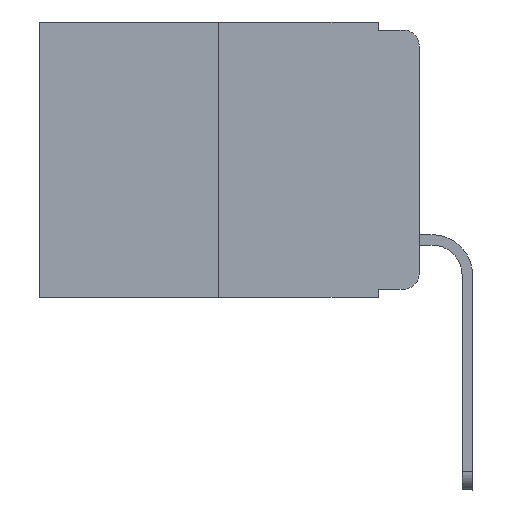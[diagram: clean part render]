
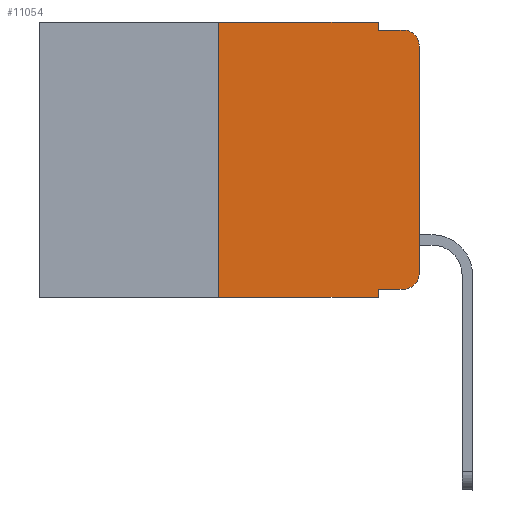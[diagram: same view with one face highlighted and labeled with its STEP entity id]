
A CAD part, left-side view. The second image highlights one B-rep face of the part: STEP entity #11054.
In plain terms, the highlighted planar face has unit normal (-1, 0, 0).
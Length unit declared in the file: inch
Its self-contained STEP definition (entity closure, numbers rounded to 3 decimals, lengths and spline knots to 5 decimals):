
#347 = CARTESIAN_POINT ( 'NONE',  ( 0., 0.051, -0.01 ) ) ;
#388 = CARTESIAN_POINT ( 'NONE',  ( 0., 0.473, 0. ) ) ;
#675 = EDGE_CURVE ( 'NONE', #12821, #10459, #7891, .T. ) ;
#1266 = CARTESIAN_POINT ( 'NONE',  ( 0., 0.051, 0. ) ) ;
#1323 = VERTEX_POINT ( 'NONE', #13808 ) ;
#1565 = DIRECTION ( 'NONE',  ( 0., -1., 0. ) ) ;
#1709 = CARTESIAN_POINT ( 'NONE',  ( 0., 0.051, 0. ) ) ;
#1970 = CARTESIAN_POINT ( 'NONE',  ( 0., 0.051, -0.01 ) ) ;
#2154 = EDGE_CURVE ( 'NONE', #12821, #5917, #11791, .T. ) ;
#2220 = DIRECTION ( 'NONE',  ( 0., 0., 1. ) ) ;
#2489 = DIRECTION ( 'NONE',  ( 0., -1., 0. ) ) ;
#2566 = DIRECTION ( 'NONE',  ( -1., 0., 0. ) ) ;
#2672 = CIRCLE ( 'NONE', #10478, 0.02 ) ;
#2825 = VECTOR ( 'NONE', #4316, 39.37008 ) ;
#2851 = VECTOR ( 'NONE', #2489, 39.37008 ) ;
#2893 = VERTEX_POINT ( 'NONE', #7720 ) ;
#2899 = CARTESIAN_POINT ( 'NONE',  ( 0., 0.25, -0.343 ) ) ;
#2956 = CIRCLE ( 'NONE', #10299, 0.02 ) ;
#3378 = CARTESIAN_POINT ( 'NONE',  ( 0., 0.25, 0. ) ) ;
#3440 = VECTOR ( 'NONE', #4258, 39.37008 ) ;
#3486 = VECTOR ( 'NONE', #8266, 39.37008 ) ;
#3659 = FACE_OUTER_BOUND ( 'NONE', #3898, .T. ) ;
#3717 = CARTESIAN_POINT ( 'NONE',  ( 0., 0.02, -0.03 ) ) ;
#3898 = EDGE_LOOP ( 'NONE', ( #11096, #4156, #4925, #9494, #6203, #8391, #6748, #5060, #5906, #5038 ) ) ;
#4055 = CARTESIAN_POINT ( 'NONE',  ( 0., 0.051, -0.333 ) ) ;
#4156 = ORIENTED_EDGE ( 'NONE', *, *, #6017, .T. ) ;
#4258 = DIRECTION ( 'NONE',  ( 0., 0., -1. ) ) ;
#4316 = DIRECTION ( 'NONE',  ( 0., -1., 0. ) ) ;
#4641 = LINE ( 'NONE', #388, #2851 ) ;
#4760 = DIRECTION ( 'NONE',  ( 0., 0., -1. ) ) ;
#4794 = DIRECTION ( 'NONE',  ( 0., 0., -1. ) ) ;
#4925 = ORIENTED_EDGE ( 'NONE', *, *, #9600, .F. ) ;
#4946 = VECTOR ( 'NONE', #1565, 39.37008 ) ;
#4984 = EDGE_CURVE ( 'NONE', #10326, #8712, #2672, .T. ) ;
#5018 = VECTOR ( 'NONE', #11070, 39.37008 ) ;
#5032 = CARTESIAN_POINT ( 'NONE',  ( 0., 0.473, -0.343 ) ) ;
#5038 = ORIENTED_EDGE ( 'NONE', *, *, #4984, .T. ) ;
#5060 = ORIENTED_EDGE ( 'NONE', *, *, #6753, .F. ) ;
#5211 = VERTEX_POINT ( 'NONE', #1709 ) ;
#5230 = CARTESIAN_POINT ( 'NONE',  ( 0., 0., 0. ) ) ;
#5351 = CARTESIAN_POINT ( 'NONE',  ( 0., 0.02, -0.313 ) ) ;
#5906 = ORIENTED_EDGE ( 'NONE', *, *, #10323, .T. ) ;
#5917 = VERTEX_POINT ( 'NONE', #8005 ) ;
#6017 = EDGE_CURVE ( 'NONE', #2893, #10927, #2956, .T. ) ;
#6203 = ORIENTED_EDGE ( 'NONE', *, *, #11391, .F. ) ;
#6416 = VECTOR ( 'NONE', #4760, 39.37008 ) ;
#6748 = ORIENTED_EDGE ( 'NONE', *, *, #2154, .T. ) ;
#6753 = EDGE_CURVE ( 'NONE', #1323, #5917, #13077, .T. ) ;
#6872 = EDGE_CURVE ( 'NONE', #5211, #7690, #12439, .T. ) ;
#6873 = DIRECTION ( 'NONE',  ( 1., 0., 0. ) ) ;
#7190 = LINE ( 'NONE', #1970, #3486 ) ;
#7275 = CARTESIAN_POINT ( 'NONE',  ( 0., 0.02, -0.333 ) ) ;
#7384 = LINE ( 'NONE', #5230, #10668 ) ;
#7690 = VERTEX_POINT ( 'NONE', #347 ) ;
#7720 = CARTESIAN_POINT ( 'NONE',  ( 0., 0., -0.03 ) ) ;
#7891 = LINE ( 'NONE', #13551, #5018 ) ;
#8005 = CARTESIAN_POINT ( 'NONE',  ( 0., 0.051, -0.343 ) ) ;
#8129 = CARTESIAN_POINT ( 'NONE',  ( 0., 0.051, 0. ) ) ;
#8266 = DIRECTION ( 'NONE',  ( 0., -1., 0. ) ) ;
#8391 = ORIENTED_EDGE ( 'NONE', *, *, #675, .F. ) ;
#8712 = VERTEX_POINT ( 'NONE', #12543 ) ;
#9049 = PLANE ( 'NONE',  #13811 ) ;
#9090 = DIRECTION ( 'NONE',  ( -1., 0., 0. ) ) ;
#9494 = ORIENTED_EDGE ( 'NONE', *, *, #6872, .F. ) ;
#9600 = EDGE_CURVE ( 'NONE', #7690, #10927, #7190, .T. ) ;
#10090 = DIRECTION ( 'NONE',  ( 0., 0., -1. ) ) ;
#10129 = DIRECTION ( 'NONE',  ( 0., 0., -1. ) ) ;
#10299 = AXIS2_PLACEMENT_3D ( 'NONE', #3717, #2566, #4794 ) ;
#10323 = EDGE_CURVE ( 'NONE', #1323, #10326, #13850, .T. ) ;
#10326 = VERTEX_POINT ( 'NONE', #7275 ) ;
#10459 = VERTEX_POINT ( 'NONE', #3378 ) ;
#10478 = AXIS2_PLACEMENT_3D ( 'NONE', #5351, #9090, #10090 ) ;
#10668 = VECTOR ( 'NONE', #2220, 39.37008 ) ;
#10927 = VERTEX_POINT ( 'NONE', #13129 ) ;
#11054 = ADVANCED_FACE ( 'NONE', ( #3659 ), #9049, .F. ) ;
#11070 = DIRECTION ( 'NONE',  ( 0., 0., 1. ) ) ;
#11096 = ORIENTED_EDGE ( 'NONE', *, *, #13478, .T. ) ;
#11391 = EDGE_CURVE ( 'NONE', #10459, #5211, #4641, .T. ) ;
#11791 = LINE ( 'NONE', #5032, #4946 ) ;
#12439 = LINE ( 'NONE', #8129, #6416 ) ;
#12543 = CARTESIAN_POINT ( 'NONE',  ( 0., 0., -0.313 ) ) ;
#12821 = VERTEX_POINT ( 'NONE', #2899 ) ;
#13077 = LINE ( 'NONE', #1266, #3440 ) ;
#13129 = CARTESIAN_POINT ( 'NONE',  ( 0., 0.02, -0.01 ) ) ;
#13478 = EDGE_CURVE ( 'NONE', #8712, #2893, #7384, .T. ) ;
#13551 = CARTESIAN_POINT ( 'NONE',  ( 0., 0.25, 0. ) ) ;
#13610 = CARTESIAN_POINT ( 'NONE',  ( 0., 0.473, 0. ) ) ;
#13808 = CARTESIAN_POINT ( 'NONE',  ( 0., 0.051, -0.333 ) ) ;
#13811 = AXIS2_PLACEMENT_3D ( 'NONE', #13610, #6873, #10129 ) ;
#13850 = LINE ( 'NONE', #4055, #2825 ) ;
